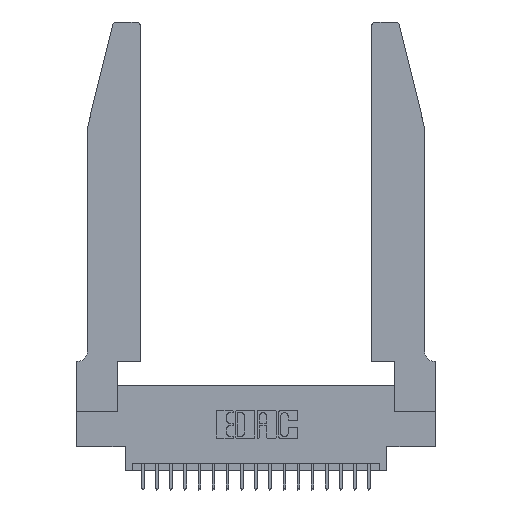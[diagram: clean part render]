
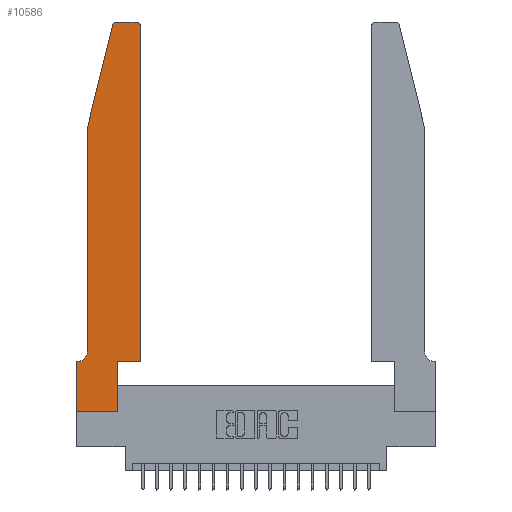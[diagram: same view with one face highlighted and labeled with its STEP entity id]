
A CAD part, top view. The second image highlights one B-rep face of the part: STEP entity #10586.
In plain terms, the highlighted planar face has unit normal (0, 0, 1).
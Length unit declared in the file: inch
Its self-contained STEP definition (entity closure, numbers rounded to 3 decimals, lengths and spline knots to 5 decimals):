
#147 = CARTESIAN_POINT ( 'NONE',  ( 0.0755, 2., 0.37 ) ) ;
#397 = VECTOR ( 'NONE', #1998, 39.37008 ) ;
#902 = CARTESIAN_POINT ( 'NONE',  ( 0.284, 2.72, 0.37 ) ) ;
#999 = ORIENTED_EDGE ( 'NONE', *, *, #2445, .T. ) ;
#1074 = CARTESIAN_POINT ( 'NONE',  ( 0., 0., 0.37 ) ) ;
#1234 = DIRECTION ( 'NONE',  ( 0., 0., 1. ) ) ;
#1452 = DIRECTION ( 'NONE',  ( 0., 0., 1. ) ) ;
#1568 = CARTESIAN_POINT ( 'NONE',  ( 0.2865, 0.35, 0.37 ) ) ;
#1998 = DIRECTION ( 'NONE',  ( 0., 1., 0. ) ) ;
#2204 = CARTESIAN_POINT ( 'NONE',  ( 0.0755, 2., 0.37 ) ) ;
#2292 = CARTESIAN_POINT ( 'NONE',  ( 0.25487, 2.72718, 0.37 ) ) ;
#2406 = LINE ( 'NONE', #2204, #14787 ) ;
#2445 = EDGE_CURVE ( 'NONE', #17701, #19198, #16124, .T. ) ;
#2830 = EDGE_CURVE ( 'NONE', #14745, #16053, #15196, .T. ) ;
#3111 = VERTEX_POINT ( 'NONE', #2292 ) ;
#3324 = ORIENTED_EDGE ( 'NONE', *, *, #10851, .T. ) ;
#3892 = LINE ( 'NONE', #13802, #12102 ) ;
#4066 = CARTESIAN_POINT ( 'NONE',  ( 0.0055, 0.35, 0.37 ) ) ;
#4195 = AXIS2_PLACEMENT_3D ( 'NONE', #17691, #1452, #4611 ) ;
#4331 = VECTOR ( 'NONE', #10258, 39.37008 ) ;
#4556 = CARTESIAN_POINT ( 'NONE',  ( 0., 0., 0.37 ) ) ;
#4611 = DIRECTION ( 'NONE',  ( 1., 0., 0. ) ) ;
#4911 = AXIS2_PLACEMENT_3D ( 'NONE', #16370, #14733, #21409 ) ;
#4996 = CARTESIAN_POINT ( 'NONE',  ( 0.0755, 0.35, 0.37 ) ) ;
#5112 = EDGE_CURVE ( 'NONE', #15708, #7566, #3892, .T. ) ;
#6055 = VERTEX_POINT ( 'NONE', #11638 ) ;
#6354 = AXIS2_PLACEMENT_3D ( 'NONE', #902, #1234, #14548 ) ;
#6491 = CARTESIAN_POINT ( 'NONE',  ( 0.0055, 0.42, 0.37 ) ) ;
#6581 = LINE ( 'NONE', #10024, #13007 ) ;
#6734 = VECTOR ( 'NONE', #7751, 39.37008 ) ;
#6802 = DIRECTION ( 'NONE',  ( -1., 0., 0. ) ) ;
#6850 = DIRECTION ( 'NONE',  ( 1., 0., 0. ) ) ;
#7566 = VERTEX_POINT ( 'NONE', #17530 ) ;
#7751 = DIRECTION ( 'NONE',  ( 0., -1., 0. ) ) ;
#7763 = CARTESIAN_POINT ( 'NONE',  ( 0.2865, 0.35, 0.37 ) ) ;
#8271 = DIRECTION ( 'NONE',  ( 0., 0., -1. ) ) ;
#8371 = DIRECTION ( 'NONE',  ( 1., 0., 0. ) ) ;
#8652 = EDGE_CURVE ( 'NONE', #14964, #6055, #6581, .T. ) ;
#8986 = EDGE_CURVE ( 'NONE', #9597, #17701, #19641, .T. ) ;
#9122 = DIRECTION ( 'NONE',  ( -0.239, -0.971, 0. ) ) ;
#9174 = CARTESIAN_POINT ( 'NONE',  ( 0.0755, 0.42, 0.37 ) ) ;
#9407 = ORIENTED_EDGE ( 'NONE', *, *, #8652, .T. ) ;
#9517 = VECTOR ( 'NONE', #20067, 39.37008 ) ;
#9597 = VERTEX_POINT ( 'NONE', #4066 ) ;
#9630 = ORIENTED_EDGE ( 'NONE', *, *, #2830, .T. ) ;
#9710 = CARTESIAN_POINT ( 'NONE',  ( 0., 0., 0.37 ) ) ;
#9855 = CIRCLE ( 'NONE', #4911, 0.03 ) ;
#10024 = CARTESIAN_POINT ( 'NONE',  ( 0.2605, 2.75, 0.37 ) ) ;
#10258 = DIRECTION ( 'NONE',  ( 0., 1., 0. ) ) ;
#10586 = ADVANCED_FACE ( 'NONE', ( #19775 ), #19555, .T. ) ;
#10851 = EDGE_CURVE ( 'NONE', #3111, #14745, #2406, .T. ) ;
#11075 = EDGE_CURVE ( 'NONE', #12346, #14964, #9855, .T. ) ;
#11359 = LINE ( 'NONE', #9710, #13038 ) ;
#11638 = CARTESIAN_POINT ( 'NONE',  ( 0.284, 2.75, 0.37 ) ) ;
#12102 = VECTOR ( 'NONE', #6850, 39.37008 ) ;
#12346 = VERTEX_POINT ( 'NONE', #20061 ) ;
#13007 = VECTOR ( 'NONE', #6802, 39.37008 ) ;
#13038 = VECTOR ( 'NONE', #8371, 39.37008 ) ;
#13223 = DIRECTION ( 'NONE',  ( -1., 0., 0. ) ) ;
#13323 = LINE ( 'NONE', #17048, #4331 ) ;
#13802 = CARTESIAN_POINT ( 'NONE',  ( 0.4505, 0.35, 0.37 ) ) ;
#14548 = DIRECTION ( 'NONE',  ( 1., 0., 0. ) ) ;
#14733 = DIRECTION ( 'NONE',  ( 0., 0., 1. ) ) ;
#14745 = VERTEX_POINT ( 'NONE', #15302 ) ;
#14787 = VECTOR ( 'NONE', #9122, 39.37008 ) ;
#14829 = ORIENTED_EDGE ( 'NONE', *, *, #20574, .T. ) ;
#14886 = EDGE_CURVE ( 'NONE', #18402, #15708, #17035, .T. ) ;
#14964 = VERTEX_POINT ( 'NONE', #15612 ) ;
#15196 = LINE ( 'NONE', #147, #20089 ) ;
#15256 = EDGE_CURVE ( 'NONE', #16053, #9597, #17941, .T. ) ;
#15288 = EDGE_CURVE ( 'NONE', #19198, #18402, #11359, .T. ) ;
#15302 = CARTESIAN_POINT ( 'NONE',  ( 0.0755, 2., 0.37 ) ) ;
#15584 = CARTESIAN_POINT ( 'NONE',  ( 0.2865, 0., 0.37 ) ) ;
#15612 = CARTESIAN_POINT ( 'NONE',  ( 0.4205, 2.75, 0.37 ) ) ;
#15629 = ORIENTED_EDGE ( 'NONE', *, *, #14886, .T. ) ;
#15708 = VERTEX_POINT ( 'NONE', #7763 ) ;
#16053 = VERTEX_POINT ( 'NONE', #9174 ) ;
#16124 = LINE ( 'NONE', #1074, #6734 ) ;
#16370 = CARTESIAN_POINT ( 'NONE',  ( 0.4205, 2.72, 0.37 ) ) ;
#16947 = ORIENTED_EDGE ( 'NONE', *, *, #8986, .T. ) ;
#17035 = LINE ( 'NONE', #1568, #397 ) ;
#17048 = CARTESIAN_POINT ( 'NONE',  ( 0.4505, 0.35, 0.37 ) ) ;
#17145 = ORIENTED_EDGE ( 'NONE', *, *, #15288, .T. ) ;
#17171 = ORIENTED_EDGE ( 'NONE', *, *, #11075, .T. ) ;
#17261 = CIRCLE ( 'NONE', #6354, 0.03 ) ;
#17514 = ORIENTED_EDGE ( 'NONE', *, *, #5112, .T. ) ;
#17530 = CARTESIAN_POINT ( 'NONE',  ( 0.4505, 0.35, 0.37 ) ) ;
#17577 = CARTESIAN_POINT ( 'NONE',  ( 0., 0.35, 0.37 ) ) ;
#17691 = CARTESIAN_POINT ( 'NONE',  ( 0., 0.35, 0.37 ) ) ;
#17701 = VERTEX_POINT ( 'NONE', #17577 ) ;
#17749 = EDGE_CURVE ( 'NONE', #6055, #3111, #17261, .T. ) ;
#17941 = CIRCLE ( 'NONE', #20386, 0.07 ) ;
#18118 = EDGE_LOOP ( 'NONE', ( #9407, #20729, #3324, #9630, #19355, #16947, #999, #17145, #15629, #17514, #14829, #17171 ) ) ;
#18402 = VERTEX_POINT ( 'NONE', #15584 ) ;
#19198 = VERTEX_POINT ( 'NONE', #4556 ) ;
#19355 = ORIENTED_EDGE ( 'NONE', *, *, #15256, .T. ) ;
#19555 = PLANE ( 'NONE',  #4195 ) ;
#19641 = LINE ( 'NONE', #4996, #9517 ) ;
#19775 = FACE_OUTER_BOUND ( 'NONE', #18118, .T. ) ;
#20061 = CARTESIAN_POINT ( 'NONE',  ( 0.4505, 2.72, 0.37 ) ) ;
#20067 = DIRECTION ( 'NONE',  ( -1., 0., 0. ) ) ;
#20089 = VECTOR ( 'NONE', #20233, 39.37008 ) ;
#20233 = DIRECTION ( 'NONE',  ( 0., -1., 0. ) ) ;
#20386 = AXIS2_PLACEMENT_3D ( 'NONE', #6491, #8271, #13223 ) ;
#20574 = EDGE_CURVE ( 'NONE', #7566, #12346, #13323, .T. ) ;
#20729 = ORIENTED_EDGE ( 'NONE', *, *, #17749, .T. ) ;
#21409 = DIRECTION ( 'NONE',  ( 1., 0., 0. ) ) ;
